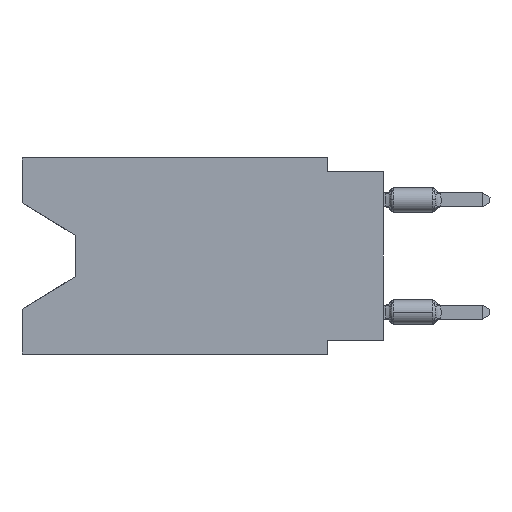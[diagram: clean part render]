
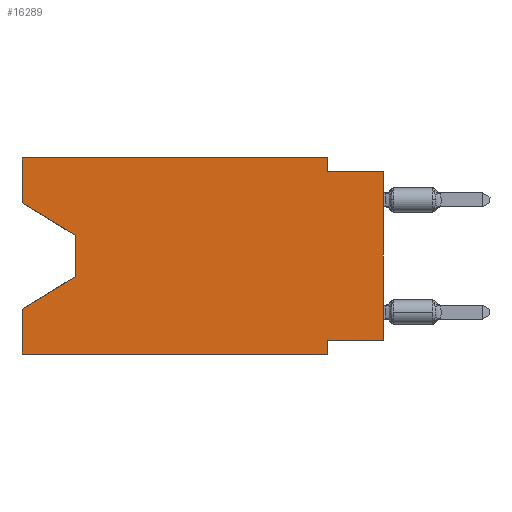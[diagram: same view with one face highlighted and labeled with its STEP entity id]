
A CAD part, left-side view. The second image highlights one B-rep face of the part: STEP entity #16289.
In plain terms, the highlighted planar face has unit normal (-1, 0, 0).
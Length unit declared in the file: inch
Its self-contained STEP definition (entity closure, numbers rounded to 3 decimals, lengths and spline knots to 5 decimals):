
#84 = ORIENTED_EDGE ( 'NONE', *, *, #10828, .T. ) ;
#440 = DIRECTION ( 'NONE',  ( 0., 0., 1. ) ) ;
#467 = LINE ( 'NONE', #7440, #5568 ) ;
#516 = VECTOR ( 'NONE', #6794, 39.37008 ) ;
#696 = CARTESIAN_POINT ( 'NONE',  ( 0., 0.55, -0.138 ) ) ;
#1009 = VERTEX_POINT ( 'NONE', #13751 ) ;
#1069 = VECTOR ( 'NONE', #14938, 39.37008 ) ;
#1241 = EDGE_CURVE ( 'NONE', #2607, #13721, #4847, .T. ) ;
#1395 = ORIENTED_EDGE ( 'NONE', *, *, #6356, .T. ) ;
#1412 = EDGE_CURVE ( 'NONE', #9310, #3242, #3518, .T. ) ;
#1541 = CARTESIAN_POINT ( 'NONE',  ( 0., 0.645, -0.08025 ) ) ;
#1964 = AXIS2_PLACEMENT_3D ( 'NONE', #8997, #2383, #4946 ) ;
#2067 = CARTESIAN_POINT ( 'NONE',  ( 0., 0.1, 0. ) ) ;
#2383 = DIRECTION ( 'NONE',  ( 1., 0., 0. ) ) ;
#2430 = CARTESIAN_POINT ( 'NONE',  ( 0., 0., -0.025 ) ) ;
#2607 = VERTEX_POINT ( 'NONE', #1541 ) ;
#3068 = ORIENTED_EDGE ( 'NONE', *, *, #6535, .T. ) ;
#3180 = VERTEX_POINT ( 'NONE', #2430 ) ;
#3242 = VERTEX_POINT ( 'NONE', #13106 ) ;
#3518 = LINE ( 'NONE', #696, #6734 ) ;
#3593 = VERTEX_POINT ( 'NONE', #16516 ) ;
#3803 = LINE ( 'NONE', #10157, #14692 ) ;
#4010 = ORIENTED_EDGE ( 'NONE', *, *, #4708, .F. ) ;
#4440 = CARTESIAN_POINT ( 'NONE',  ( 0., 0., -0.025 ) ) ;
#4708 = EDGE_CURVE ( 'NONE', #3593, #3180, #8077, .T. ) ;
#4847 = LINE ( 'NONE', #6365, #15468 ) ;
#4915 = DIRECTION ( 'NONE',  ( 0., -1., 0. ) ) ;
#4946 = DIRECTION ( 'NONE',  ( 0., 0., -1. ) ) ;
#5568 = VECTOR ( 'NONE', #8794, 39.37008 ) ;
#5650 = LINE ( 'NONE', #6834, #16518 ) ;
#6066 = DIRECTION ( 'NONE',  ( 0., 0., -1. ) ) ;
#6114 = LINE ( 'NONE', #14007, #13642 ) ;
#6275 = ORIENTED_EDGE ( 'NONE', *, *, #7364, .F. ) ;
#6356 = EDGE_CURVE ( 'NONE', #2607, #9310, #15783, .T. ) ;
#6365 = CARTESIAN_POINT ( 'NONE',  ( 0., 0.645, 0. ) ) ;
#6535 = EDGE_CURVE ( 'NONE', #3242, #8893, #13309, .T. ) ;
#6710 = ORIENTED_EDGE ( 'NONE', *, *, #12276, .F. ) ;
#6734 = VECTOR ( 'NONE', #16328, 39.37008 ) ;
#6794 = DIRECTION ( 'NONE',  ( 0., -0.855, -0.519 ) ) ;
#6834 = CARTESIAN_POINT ( 'NONE',  ( 0., 0.645, 0. ) ) ;
#7085 = ORIENTED_EDGE ( 'NONE', *, *, #13897, .F. ) ;
#7196 = CARTESIAN_POINT ( 'NONE',  ( 0., 0.645, -0.35 ) ) ;
#7230 = VECTOR ( 'NONE', #6066, 39.37008 ) ;
#7313 = ORIENTED_EDGE ( 'NONE', *, *, #16690, .T. ) ;
#7364 = EDGE_CURVE ( 'NONE', #11876, #8893, #5650, .T. ) ;
#7440 = CARTESIAN_POINT ( 'NONE',  ( 0., 0., -0.325 ) ) ;
#7461 = DIRECTION ( 'NONE',  ( 0., 0., 1. ) ) ;
#7485 = PLANE ( 'NONE',  #1964 ) ;
#7681 = ORIENTED_EDGE ( 'NONE', *, *, #1241, .F. ) ;
#7798 = CARTESIAN_POINT ( 'NONE',  ( 0., 0.645, -0.08025 ) ) ;
#7991 = ORIENTED_EDGE ( 'NONE', *, *, #8459, .F. ) ;
#8077 = LINE ( 'NONE', #4440, #11518 ) ;
#8459 = EDGE_CURVE ( 'NONE', #13721, #10184, #3803, .T. ) ;
#8499 = DIRECTION ( 'NONE',  ( 0., 0., 1. ) ) ;
#8551 = VERTEX_POINT ( 'NONE', #10242 ) ;
#8593 = VECTOR ( 'NONE', #8499, 39.37008 ) ;
#8696 = CARTESIAN_POINT ( 'NONE',  ( 0., 0.645, -0.26975 ) ) ;
#8794 = DIRECTION ( 'NONE',  ( 0., 1., 0. ) ) ;
#8893 = VERTEX_POINT ( 'NONE', #8696 ) ;
#8920 = FACE_OUTER_BOUND ( 'NONE', #11008, .T. ) ;
#8997 = CARTESIAN_POINT ( 'NONE',  ( 0., 0.645, 0. ) ) ;
#9267 = DIRECTION ( 'NONE',  ( 0., -1., 0. ) ) ;
#9310 = VERTEX_POINT ( 'NONE', #14035 ) ;
#9578 = CARTESIAN_POINT ( 'NONE',  ( 0., 0.55, -0.212 ) ) ;
#9706 = DIRECTION ( 'NONE',  ( 0., 0., -1. ) ) ;
#10004 = CARTESIAN_POINT ( 'NONE',  ( 0., 0.1, 0. ) ) ;
#10157 = CARTESIAN_POINT ( 'NONE',  ( 0., 0.645, 0. ) ) ;
#10184 = VERTEX_POINT ( 'NONE', #10004 ) ;
#10242 = CARTESIAN_POINT ( 'NONE',  ( 0., 0., -0.325 ) ) ;
#10788 = LINE ( 'NONE', #15987, #8593 ) ;
#10828 = EDGE_CURVE ( 'NONE', #8551, #3180, #10788, .T. ) ;
#10849 = ORIENTED_EDGE ( 'NONE', *, *, #12890, .F. ) ;
#11008 = EDGE_LOOP ( 'NONE', ( #1395, #11166, #3068, #6275, #7313, #6710, #10849, #84, #4010, #7085, #7991, #7681 ) ) ;
#11128 = CARTESIAN_POINT ( 'NONE',  ( 0., 0.1, -0.35 ) ) ;
#11166 = ORIENTED_EDGE ( 'NONE', *, *, #1412, .T. ) ;
#11518 = VECTOR ( 'NONE', #9267, 39.37008 ) ;
#11876 = VERTEX_POINT ( 'NONE', #7196 ) ;
#11996 = CARTESIAN_POINT ( 'NONE',  ( 0., 0.645, 0. ) ) ;
#12276 = EDGE_CURVE ( 'NONE', #1009, #13370, #15372, .T. ) ;
#12890 = EDGE_CURVE ( 'NONE', #8551, #1009, #467, .T. ) ;
#13106 = CARTESIAN_POINT ( 'NONE',  ( 0., 0.55, -0.212 ) ) ;
#13309 = LINE ( 'NONE', #9578, #1069 ) ;
#13370 = VERTEX_POINT ( 'NONE', #16251 ) ;
#13642 = VECTOR ( 'NONE', #15437, 39.37008 ) ;
#13707 = LINE ( 'NONE', #2067, #7230 ) ;
#13721 = VERTEX_POINT ( 'NONE', #11996 ) ;
#13751 = CARTESIAN_POINT ( 'NONE',  ( 0., 0.1, -0.325 ) ) ;
#13897 = EDGE_CURVE ( 'NONE', #10184, #3593, #13707, .T. ) ;
#14007 = CARTESIAN_POINT ( 'NONE',  ( 0., 0.645, -0.35 ) ) ;
#14035 = CARTESIAN_POINT ( 'NONE',  ( 0., 0.55, -0.138 ) ) ;
#14692 = VECTOR ( 'NONE', #4915, 39.37008 ) ;
#14938 = DIRECTION ( 'NONE',  ( 0., 0.855, -0.519 ) ) ;
#15364 = VECTOR ( 'NONE', #9706, 39.37008 ) ;
#15372 = LINE ( 'NONE', #11128, #15364 ) ;
#15437 = DIRECTION ( 'NONE',  ( 0., -1., 0. ) ) ;
#15468 = VECTOR ( 'NONE', #7461, 39.37008 ) ;
#15783 = LINE ( 'NONE', #7798, #516 ) ;
#15987 = CARTESIAN_POINT ( 'NONE',  ( 0., 0., 0. ) ) ;
#16251 = CARTESIAN_POINT ( 'NONE',  ( 0., 0.1, -0.35 ) ) ;
#16289 = ADVANCED_FACE ( 'NONE', ( #8920 ), #7485, .F. ) ;
#16328 = DIRECTION ( 'NONE',  ( 0., 0., -1. ) ) ;
#16516 = CARTESIAN_POINT ( 'NONE',  ( 0., 0.1, -0.025 ) ) ;
#16518 = VECTOR ( 'NONE', #440, 39.37008 ) ;
#16690 = EDGE_CURVE ( 'NONE', #11876, #13370, #6114, .T. ) ;
